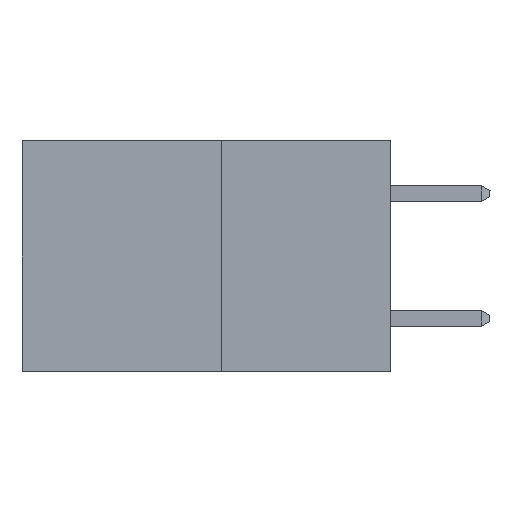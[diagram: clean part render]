
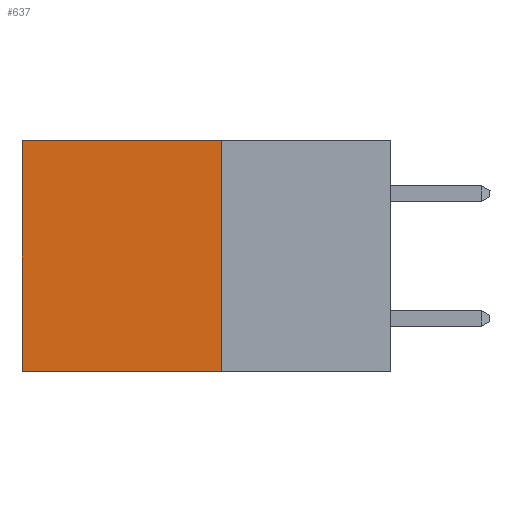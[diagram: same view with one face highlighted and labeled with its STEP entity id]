
A CAD part, left-side view. The second image highlights one B-rep face of the part: STEP entity #637.
In plain terms, the highlighted planar face has unit normal (-1, 0, 0).
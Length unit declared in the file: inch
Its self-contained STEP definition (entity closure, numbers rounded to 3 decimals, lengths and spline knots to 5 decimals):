
#394 = CARTESIAN_POINT ( 'NONE',  ( 0.277, 0.59, 0. ) ) ;
#424 = DIRECTION ( 'NONE',  ( 0., 0., -1. ) ) ;
#637 = ADVANCED_FACE ( 'NONE', ( #14854 ), #1718, .F. ) ;
#1191 = DIRECTION ( 'NONE',  ( 1., 0., 0. ) ) ;
#1238 = ORIENTED_EDGE ( 'NONE', *, *, #25616, .T. ) ;
#1469 = CARTESIAN_POINT ( 'NONE',  ( 0.277, 0.27, -0.37 ) ) ;
#1718 = PLANE ( 'NONE',  #5711 ) ;
#2068 = CARTESIAN_POINT ( 'NONE',  ( 0.277, 0.59, -0.37 ) ) ;
#3011 = ORIENTED_EDGE ( 'NONE', *, *, #15493, .F. ) ;
#3669 = VECTOR ( 'NONE', #9168, 39.37008 ) ;
#3861 = EDGE_LOOP ( 'NONE', ( #31700, #26881, #3011, #1238 ) ) ;
#4873 = CARTESIAN_POINT ( 'NONE',  ( 0.277, 0.27, -0.37 ) ) ;
#5055 = VERTEX_POINT ( 'NONE', #19612 ) ;
#5711 = AXIS2_PLACEMENT_3D ( 'NONE', #1469, #1191, #424 ) ;
#7917 = CARTESIAN_POINT ( 'NONE',  ( 0.277, 0.27, 0. ) ) ;
#9168 = DIRECTION ( 'NONE',  ( 0., 1., 0. ) ) ;
#9896 = VECTOR ( 'NONE', #27213, 39.37008 ) ;
#10662 = LINE ( 'NONE', #12538, #9896 ) ;
#12538 = CARTESIAN_POINT ( 'NONE',  ( 0.277, 0.27, -0.37 ) ) ;
#12816 = LINE ( 'NONE', #4873, #25830 ) ;
#13569 = LINE ( 'NONE', #16562, #25007 ) ;
#14106 = EDGE_CURVE ( 'NONE', #5055, #31233, #10662, .T. ) ;
#14854 = FACE_OUTER_BOUND ( 'NONE', #3861, .T. ) ;
#15493 = EDGE_CURVE ( 'NONE', #16795, #5055, #12816, .T. ) ;
#15973 = EDGE_CURVE ( 'NONE', #28337, #31233, #13569, .T. ) ;
#16562 = CARTESIAN_POINT ( 'NONE',  ( 0.277, 0.59, -0.37 ) ) ;
#16733 = LINE ( 'NONE', #21411, #3669 ) ;
#16795 = VERTEX_POINT ( 'NONE', #7917 ) ;
#19026 = DIRECTION ( 'NONE',  ( 0., 0., -1. ) ) ;
#19612 = CARTESIAN_POINT ( 'NONE',  ( 0.277, 0.27, -0.37 ) ) ;
#21411 = CARTESIAN_POINT ( 'NONE',  ( 0.277, 0.27, 0. ) ) ;
#25007 = VECTOR ( 'NONE', #19026, 39.37008 ) ;
#25616 = EDGE_CURVE ( 'NONE', #16795, #28337, #16733, .T. ) ;
#25830 = VECTOR ( 'NONE', #29379, 39.37008 ) ;
#26881 = ORIENTED_EDGE ( 'NONE', *, *, #14106, .F. ) ;
#27213 = DIRECTION ( 'NONE',  ( 0., 1., 0. ) ) ;
#28337 = VERTEX_POINT ( 'NONE', #394 ) ;
#29379 = DIRECTION ( 'NONE',  ( 0., 0., -1. ) ) ;
#31233 = VERTEX_POINT ( 'NONE', #2068 ) ;
#31700 = ORIENTED_EDGE ( 'NONE', *, *, #15973, .T. ) ;
